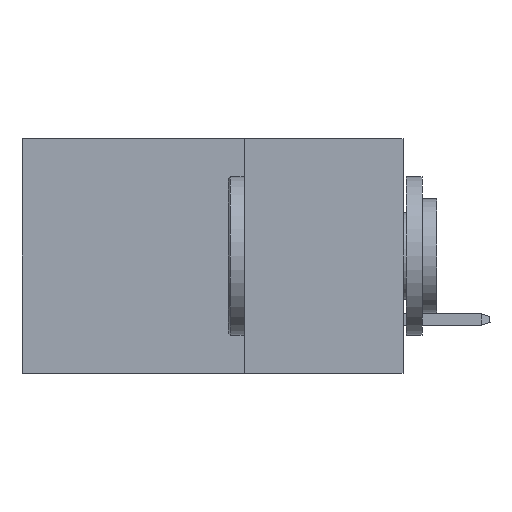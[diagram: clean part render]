
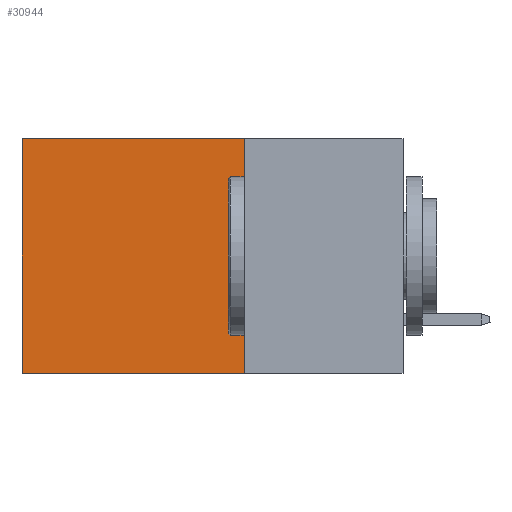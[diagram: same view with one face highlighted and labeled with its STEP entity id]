
A CAD part, left-side view. The second image highlights one B-rep face of the part: STEP entity #30944.
In plain terms, the highlighted planar face has unit normal (-1, 0, 0).
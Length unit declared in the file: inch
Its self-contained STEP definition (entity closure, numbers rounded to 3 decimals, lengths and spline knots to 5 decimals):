
#801 = PLANE ( 'NONE',  #18788 ) ;
#1410 = EDGE_CURVE ( 'NONE', #28036, #24299, #25670, .T. ) ;
#2833 = CARTESIAN_POINT ( 'NONE',  ( 0.2875, 0.25, -0.37 ) ) ;
#3013 = CARTESIAN_POINT ( 'NONE',  ( 0.2875, 0.6, 0. ) ) ;
#3604 = DIRECTION ( 'NONE',  ( 0., 1., 0. ) ) ;
#4222 = DIRECTION ( 'NONE',  ( 0., 0., -1. ) ) ;
#4825 = VECTOR ( 'NONE', #16894, 39.37008 ) ;
#6825 = LINE ( 'NONE', #35470, #39336 ) ;
#10324 = CARTESIAN_POINT ( 'NONE',  ( 0.2875, 0.25, 0. ) ) ;
#10552 = VECTOR ( 'NONE', #3604, 39.37008 ) ;
#11169 = ORIENTED_EDGE ( 'NONE', *, *, #1410, .F. ) ;
#12673 = CARTESIAN_POINT ( 'NONE',  ( 0.2875, 0.25, 0. ) ) ;
#13241 = CARTESIAN_POINT ( 'NONE',  ( 0.2875, 0.25, 0. ) ) ;
#16168 = EDGE_CURVE ( 'NONE', #28036, #33818, #35092, .T. ) ;
#16894 = DIRECTION ( 'NONE',  ( 0., 0., -1. ) ) ;
#17723 = VECTOR ( 'NONE', #24475, 39.37008 ) ;
#18319 = EDGE_CURVE ( 'NONE', #33818, #36402, #6825, .T. ) ;
#18788 = AXIS2_PLACEMENT_3D ( 'NONE', #12673, #22059, #37392 ) ;
#19335 = CARTESIAN_POINT ( 'NONE',  ( 0.2875, 0.25, -0.37 ) ) ;
#20252 = CARTESIAN_POINT ( 'NONE',  ( 0.2875, 0.25, 0. ) ) ;
#22059 = DIRECTION ( 'NONE',  ( 1., 0., 0. ) ) ;
#22248 = FACE_OUTER_BOUND ( 'NONE', #31339, .T. ) ;
#24299 = VERTEX_POINT ( 'NONE', #19335 ) ;
#24441 = ORIENTED_EDGE ( 'NONE', *, *, #24710, .F. ) ;
#24475 = DIRECTION ( 'NONE',  ( 0., 1., 0. ) ) ;
#24710 = EDGE_CURVE ( 'NONE', #24299, #36402, #30422, .T. ) ;
#25670 = LINE ( 'NONE', #13241, #4825 ) ;
#28036 = VERTEX_POINT ( 'NONE', #20252 ) ;
#30422 = LINE ( 'NONE', #2833, #17723 ) ;
#30944 = ADVANCED_FACE ( 'NONE', ( #22248 ), #801, .F. ) ;
#31339 = EDGE_LOOP ( 'NONE', ( #40187, #24441, #11169, #36341 ) ) ;
#33818 = VERTEX_POINT ( 'NONE', #3013 ) ;
#35092 = LINE ( 'NONE', #10324, #10552 ) ;
#35470 = CARTESIAN_POINT ( 'NONE',  ( 0.2875, 0.6, 0. ) ) ;
#36341 = ORIENTED_EDGE ( 'NONE', *, *, #16168, .T. ) ;
#36383 = CARTESIAN_POINT ( 'NONE',  ( 0.2875, 0.6, -0.37 ) ) ;
#36402 = VERTEX_POINT ( 'NONE', #36383 ) ;
#37392 = DIRECTION ( 'NONE',  ( 0., 0., -1. ) ) ;
#39336 = VECTOR ( 'NONE', #4222, 39.37008 ) ;
#40187 = ORIENTED_EDGE ( 'NONE', *, *, #18319, .T. ) ;
